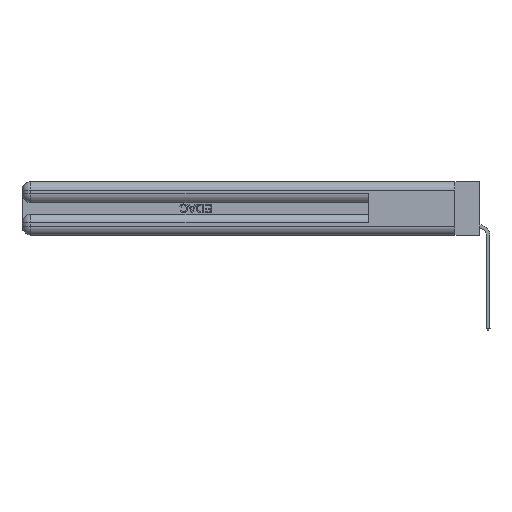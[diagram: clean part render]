
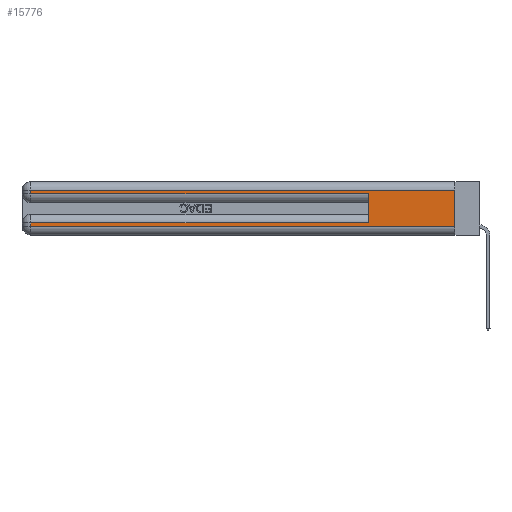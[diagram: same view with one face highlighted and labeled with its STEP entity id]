
A CAD part, left-side view. The second image highlights one B-rep face of the part: STEP entity #15776.
In plain terms, the highlighted planar face has unit normal (-1, 0, 0).
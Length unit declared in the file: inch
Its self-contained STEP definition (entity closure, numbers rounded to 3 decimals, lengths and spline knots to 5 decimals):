
#641 = DIRECTION ( 'NONE',  ( 0., -1., 0. ) ) ;
#958 = CARTESIAN_POINT ( 'NONE',  ( 0., 0., 0.085 ) ) ;
#1004 = CARTESIAN_POINT ( 'NONE',  ( 0., 2.94, 0.37 ) ) ;
#1106 = CARTESIAN_POINT ( 'NONE',  ( 0., 0., 0.37 ) ) ;
#1115 = EDGE_CURVE ( 'NONE', #34192, #8331, #14777, .T. ) ;
#1643 = CARTESIAN_POINT ( 'NONE',  ( 0., 0.6, 0.145 ) ) ;
#2266 = VERTEX_POINT ( 'NONE', #5941 ) ;
#2519 = VECTOR ( 'NONE', #12145, 39.37008 ) ;
#2631 = CARTESIAN_POINT ( 'NONE',  ( 0., 0., 0.37 ) ) ;
#5350 = FACE_OUTER_BOUND ( 'NONE', #8192, .T. ) ;
#5524 = PLANE ( 'NONE',  #23720 ) ;
#5941 = CARTESIAN_POINT ( 'NONE',  ( 0., 2.94, 0.31 ) ) ;
#6536 = LINE ( 'NONE', #1106, #2519 ) ;
#7157 = VERTEX_POINT ( 'NONE', #25757 ) ;
#7725 = VERTEX_POINT ( 'NONE', #16594 ) ;
#8192 = EDGE_LOOP ( 'NONE', ( #35651, #21752, #16360, #11466, #19130, #22420, #12451, #29244 ) ) ;
#8331 = VERTEX_POINT ( 'NONE', #30833 ) ;
#8676 = CARTESIAN_POINT ( 'NONE',  ( 0., 0., 0.31 ) ) ;
#9529 = CARTESIAN_POINT ( 'NONE',  ( 0., 0., 0.06 ) ) ;
#10328 = LINE ( 'NONE', #1643, #12967 ) ;
#11351 = EDGE_CURVE ( 'NONE', #2266, #16698, #28731, .T. ) ;
#11466 = ORIENTED_EDGE ( 'NONE', *, *, #25474, .T. ) ;
#12043 = DIRECTION ( 'NONE',  ( 0., 0., -1. ) ) ;
#12138 = EDGE_CURVE ( 'NONE', #7157, #34192, #19595, .T. ) ;
#12145 = DIRECTION ( 'NONE',  ( 0., 0., -1. ) ) ;
#12451 = ORIENTED_EDGE ( 'NONE', *, *, #1115, .T. ) ;
#12496 = VECTOR ( 'NONE', #641, 39.37008 ) ;
#12967 = VECTOR ( 'NONE', #32416, 39.37008 ) ;
#13903 = VERTEX_POINT ( 'NONE', #15205 ) ;
#14777 = LINE ( 'NONE', #1004, #32169 ) ;
#15205 = CARTESIAN_POINT ( 'NONE',  ( 0., 0.6, 0.285 ) ) ;
#15776 = ADVANCED_FACE ( 'NONE', ( #5350 ), #5524, .F. ) ;
#15842 = CARTESIAN_POINT ( 'NONE',  ( 0., 0., 0.285 ) ) ;
#16360 = ORIENTED_EDGE ( 'NONE', *, *, #11351, .T. ) ;
#16366 = LINE ( 'NONE', #15842, #25730 ) ;
#16594 = CARTESIAN_POINT ( 'NONE',  ( 0., 0., 0.31 ) ) ;
#16698 = VERTEX_POINT ( 'NONE', #17588 ) ;
#16760 = DIRECTION ( 'NONE',  ( 1., 0., 0. ) ) ;
#16904 = DIRECTION ( 'NONE',  ( 0., 1., 0. ) ) ;
#17588 = CARTESIAN_POINT ( 'NONE',  ( 0., 2.94, 0.285 ) ) ;
#17785 = VERTEX_POINT ( 'NONE', #9529 ) ;
#19130 = ORIENTED_EDGE ( 'NONE', *, *, #22273, .F. ) ;
#19595 = LINE ( 'NONE', #958, #20814 ) ;
#19891 = DIRECTION ( 'NONE',  ( 0., 1., 0. ) ) ;
#20814 = VECTOR ( 'NONE', #16904, 39.37008 ) ;
#21021 = VECTOR ( 'NONE', #25293, 39.37008 ) ;
#21752 = ORIENTED_EDGE ( 'NONE', *, *, #30736, .T. ) ;
#21814 = DIRECTION ( 'NONE',  ( 0., 0., -1. ) ) ;
#22149 = EDGE_CURVE ( 'NONE', #7725, #17785, #6536, .T. ) ;
#22273 = EDGE_CURVE ( 'NONE', #7157, #13903, #10328, .T. ) ;
#22420 = ORIENTED_EDGE ( 'NONE', *, *, #12138, .T. ) ;
#23720 = AXIS2_PLACEMENT_3D ( 'NONE', #2631, #16760, #21814 ) ;
#24654 = VECTOR ( 'NONE', #19891, 39.37008 ) ;
#25293 = DIRECTION ( 'NONE',  ( 0., 0., -1. ) ) ;
#25319 = LINE ( 'NONE', #8676, #24654 ) ;
#25434 = LINE ( 'NONE', #27801, #12496 ) ;
#25474 = EDGE_CURVE ( 'NONE', #16698, #13903, #16366, .T. ) ;
#25730 = VECTOR ( 'NONE', #27393, 39.37008 ) ;
#25757 = CARTESIAN_POINT ( 'NONE',  ( 0., 0.6, 0.085 ) ) ;
#25975 = CARTESIAN_POINT ( 'NONE',  ( 0., 2.94, 0.085 ) ) ;
#26416 = EDGE_CURVE ( 'NONE', #8331, #17785, #25434, .T. ) ;
#27393 = DIRECTION ( 'NONE',  ( 0., -1., 0. ) ) ;
#27801 = CARTESIAN_POINT ( 'NONE',  ( 0., 0., 0.06 ) ) ;
#28551 = CARTESIAN_POINT ( 'NONE',  ( 0., 2.94, 0.37 ) ) ;
#28731 = LINE ( 'NONE', #28551, #21021 ) ;
#29244 = ORIENTED_EDGE ( 'NONE', *, *, #26416, .T. ) ;
#30736 = EDGE_CURVE ( 'NONE', #7725, #2266, #25319, .T. ) ;
#30833 = CARTESIAN_POINT ( 'NONE',  ( 0., 2.94, 0.06 ) ) ;
#32169 = VECTOR ( 'NONE', #12043, 39.37008 ) ;
#32416 = DIRECTION ( 'NONE',  ( 0., 0., 1. ) ) ;
#34192 = VERTEX_POINT ( 'NONE', #25975 ) ;
#35651 = ORIENTED_EDGE ( 'NONE', *, *, #22149, .F. ) ;
